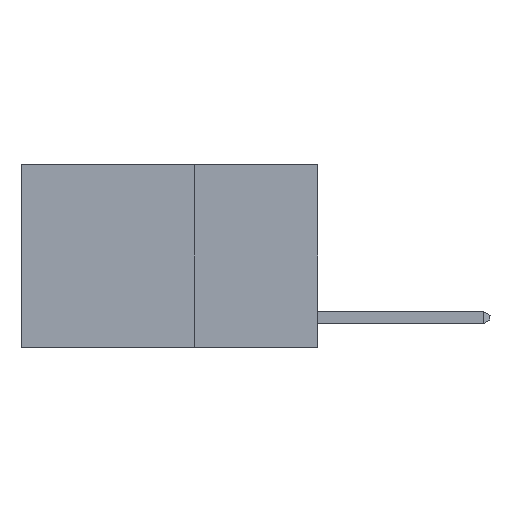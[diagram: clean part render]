
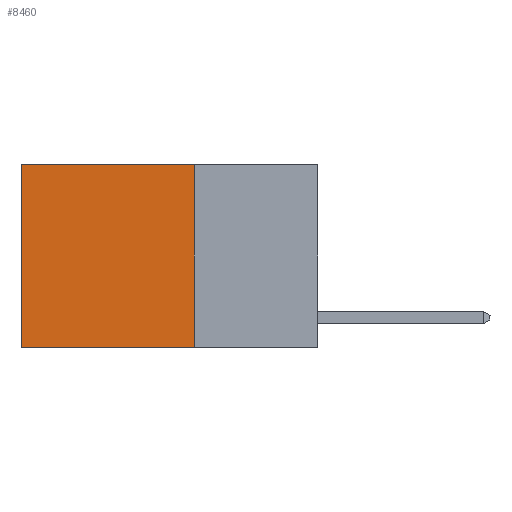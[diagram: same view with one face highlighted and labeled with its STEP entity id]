
A CAD part, left-side view. The second image highlights one B-rep face of the part: STEP entity #8460.
In plain terms, the highlighted planar face has unit normal (-1, 0, 0).
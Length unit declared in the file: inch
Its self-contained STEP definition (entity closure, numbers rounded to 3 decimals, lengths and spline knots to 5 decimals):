
#626 = LINE ( 'NONE', #6770, #10503 ) ;
#850 = FACE_OUTER_BOUND ( 'NONE', #10816, .T. ) ;
#1125 = CARTESIAN_POINT ( 'NONE',  ( 0.2625, 0.25, 0. ) ) ;
#1690 = VECTOR ( 'NONE', #2692, 39.37008 ) ;
#1952 = LINE ( 'NONE', #4379, #1690 ) ;
#2692 = DIRECTION ( 'NONE',  ( 0., 0., -1. ) ) ;
#2738 = DIRECTION ( 'NONE',  ( 0., 1., 0. ) ) ;
#3587 = VECTOR ( 'NONE', #21516, 39.37008 ) ;
#3775 = AXIS2_PLACEMENT_3D ( 'NONE', #5464, #16527, #6106 ) ;
#4106 = ORIENTED_EDGE ( 'NONE', *, *, #12016, .F. ) ;
#4379 = CARTESIAN_POINT ( 'NONE',  ( 0.2625, 0.6, 0. ) ) ;
#5464 = CARTESIAN_POINT ( 'NONE',  ( 0.2625, 0.25, 0. ) ) ;
#6106 = DIRECTION ( 'NONE',  ( 0., 0., -1. ) ) ;
#6770 = CARTESIAN_POINT ( 'NONE',  ( 0.2625, 0.25, 0. ) ) ;
#8189 = LINE ( 'NONE', #1125, #19704 ) ;
#8460 = ADVANCED_FACE ( 'NONE', ( #850 ), #21162, .F. ) ;
#10231 = EDGE_CURVE ( 'NONE', #16113, #15848, #1952, .T. ) ;
#10246 = ORIENTED_EDGE ( 'NONE', *, *, #22062, .F. ) ;
#10370 = CARTESIAN_POINT ( 'NONE',  ( 0.2625, 0.25, 0. ) ) ;
#10503 = VECTOR ( 'NONE', #20797, 39.37008 ) ;
#10816 = EDGE_LOOP ( 'NONE', ( #14713, #4106, #10246, #19936 ) ) ;
#12016 = EDGE_CURVE ( 'NONE', #20105, #15848, #14253, .T. ) ;
#14253 = LINE ( 'NONE', #14624, #3587 ) ;
#14624 = CARTESIAN_POINT ( 'NONE',  ( 0.2625, 0.25, -0.37 ) ) ;
#14713 = ORIENTED_EDGE ( 'NONE', *, *, #10231, .T. ) ;
#15848 = VERTEX_POINT ( 'NONE', #20248 ) ;
#16113 = VERTEX_POINT ( 'NONE', #20535 ) ;
#16527 = DIRECTION ( 'NONE',  ( 1., 0., 0. ) ) ;
#19704 = VECTOR ( 'NONE', #2738, 39.37008 ) ;
#19936 = ORIENTED_EDGE ( 'NONE', *, *, #20042, .T. ) ;
#20042 = EDGE_CURVE ( 'NONE', #22314, #16113, #8189, .T. ) ;
#20105 = VERTEX_POINT ( 'NONE', #21885 ) ;
#20248 = CARTESIAN_POINT ( 'NONE',  ( 0.2625, 0.6, -0.37 ) ) ;
#20535 = CARTESIAN_POINT ( 'NONE',  ( 0.2625, 0.6, 0. ) ) ;
#20797 = DIRECTION ( 'NONE',  ( 0., 0., -1. ) ) ;
#21162 = PLANE ( 'NONE',  #3775 ) ;
#21516 = DIRECTION ( 'NONE',  ( 0., 1., 0. ) ) ;
#21885 = CARTESIAN_POINT ( 'NONE',  ( 0.2625, 0.25, -0.37 ) ) ;
#22062 = EDGE_CURVE ( 'NONE', #22314, #20105, #626, .T. ) ;
#22314 = VERTEX_POINT ( 'NONE', #10370 ) ;
